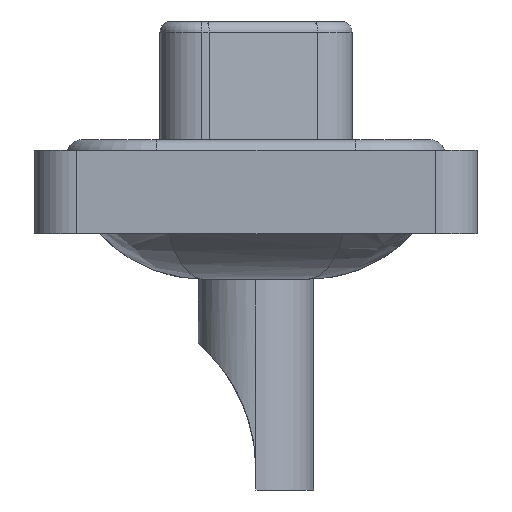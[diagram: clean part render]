
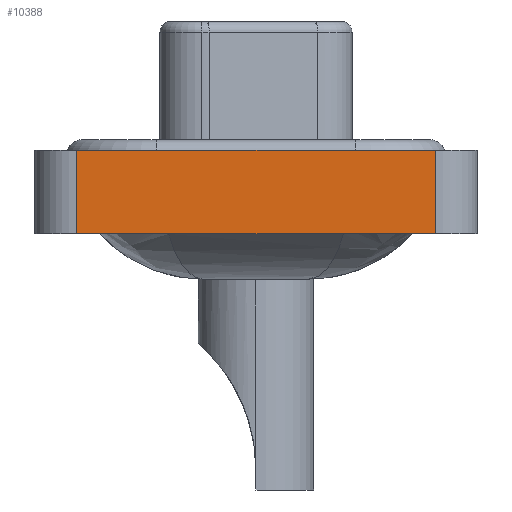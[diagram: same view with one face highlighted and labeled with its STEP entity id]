
A CAD part, left-side view. The second image highlights one B-rep face of the part: STEP entity #10388.
In plain terms, the highlighted planar face has unit normal (-1, 0, 0).
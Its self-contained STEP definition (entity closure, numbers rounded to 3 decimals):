
#737 = VECTOR ( 'NONE', #13289, 1000. ) ;
#774 = CARTESIAN_POINT ( 'NONE',  ( -7.35, -8.55, -3.6 ) ) ;
#922 = LINE ( 'NONE', #2098, #7154 ) ;
#2098 = CARTESIAN_POINT ( 'NONE',  ( -7.35, -8.55, -3.6 ) ) ;
#2918 = VECTOR ( 'NONE', #20541, 1000. ) ;
#3524 = EDGE_LOOP ( 'NONE', ( #11521, #11682, #3740, #15401 ) ) ;
#3740 = ORIENTED_EDGE ( 'NONE', *, *, #20737, .F. ) ;
#3886 = CARTESIAN_POINT ( 'NONE',  ( -7.35, -8.55, -3.6 ) ) ;
#4817 = CARTESIAN_POINT ( 'NONE',  ( -7.35, -8.55, 0.4 ) ) ;
#4917 = EDGE_CURVE ( 'NONE', #15471, #16793, #20853, .T. ) ;
#5242 = CARTESIAN_POINT ( 'NONE',  ( -7.35, -8.55, -3.6 ) ) ;
#6393 = CARTESIAN_POINT ( 'NONE',  ( -7.35, 8.55, 0.4 ) ) ;
#7154 = VECTOR ( 'NONE', #15046, 1000. ) ;
#7248 = DIRECTION ( 'NONE',  ( 0., 0., 1. ) ) ;
#7960 = LINE ( 'NONE', #16342, #16874 ) ;
#9515 = VERTEX_POINT ( 'NONE', #16990 ) ;
#9983 = EDGE_CURVE ( 'NONE', #14854, #16793, #922, .T. ) ;
#10388 = ADVANCED_FACE ( 'NONE', ( #18710 ), #15323, .T. ) ;
#11141 = DIRECTION ( 'NONE',  ( 0., 0., 1. ) ) ;
#11521 = ORIENTED_EDGE ( 'NONE', *, *, #9983, .T. ) ;
#11682 = ORIENTED_EDGE ( 'NONE', *, *, #4917, .F. ) ;
#11914 = LINE ( 'NONE', #5242, #737 ) ;
#11973 = EDGE_CURVE ( 'NONE', #9515, #14854, #11914, .T. ) ;
#12574 = AXIS2_PLACEMENT_3D ( 'NONE', #774, #15413, #7248 ) ;
#13289 = DIRECTION ( 'NONE',  ( 0., -1., 0. ) ) ;
#14854 = VERTEX_POINT ( 'NONE', #3886 ) ;
#15046 = DIRECTION ( 'NONE',  ( 0., 0., 1. ) ) ;
#15323 = PLANE ( 'NONE',  #12574 ) ;
#15401 = ORIENTED_EDGE ( 'NONE', *, *, #11973, .T. ) ;
#15413 = DIRECTION ( 'NONE',  ( -1., 0., 0. ) ) ;
#15471 = VERTEX_POINT ( 'NONE', #6393 ) ;
#16342 = CARTESIAN_POINT ( 'NONE',  ( -7.35, 8.55, -3.6 ) ) ;
#16793 = VERTEX_POINT ( 'NONE', #4817 ) ;
#16874 = VECTOR ( 'NONE', #11141, 1000. ) ;
#16990 = CARTESIAN_POINT ( 'NONE',  ( -7.35, 8.55, -3.6 ) ) ;
#18710 = FACE_OUTER_BOUND ( 'NONE', #3524, .T. ) ;
#20541 = DIRECTION ( 'NONE',  ( 0., -1., 0. ) ) ;
#20656 = CARTESIAN_POINT ( 'NONE',  ( -7.35, -8.55, 0.4 ) ) ;
#20737 = EDGE_CURVE ( 'NONE', #9515, #15471, #7960, .T. ) ;
#20853 = LINE ( 'NONE', #20656, #2918 ) ;
